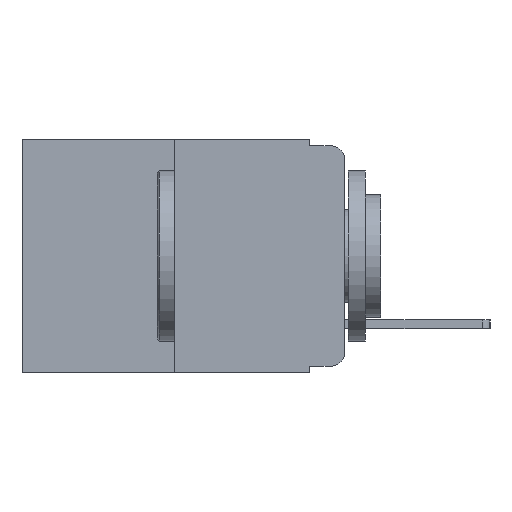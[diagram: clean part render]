
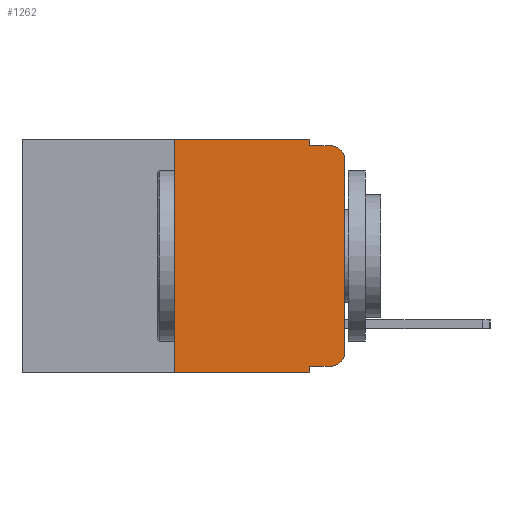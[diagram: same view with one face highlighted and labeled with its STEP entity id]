
A CAD part, left-side view. The second image highlights one B-rep face of the part: STEP entity #1262.
In plain terms, the highlighted planar face has unit normal (-1, 0, 0).
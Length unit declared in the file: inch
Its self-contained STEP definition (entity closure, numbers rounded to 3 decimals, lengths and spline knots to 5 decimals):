
#20 = CARTESIAN_POINT ( 'NONE',  ( 0., 0.02, -0.313 ) ) ;
#43 = CARTESIAN_POINT ( 'NONE',  ( 0., 0.473, 0. ) ) ;
#132 = DIRECTION ( 'NONE',  ( 0., 0., -1. ) ) ;
#146 = DIRECTION ( 'NONE',  ( -1., 0., 0. ) ) ;
#614 = VERTEX_POINT ( 'NONE', #5338 ) ;
#762 = VECTOR ( 'NONE', #6290, 39.37008 ) ;
#983 = DIRECTION ( 'NONE',  ( 1., 0., 0. ) ) ;
#1009 = DIRECTION ( 'NONE',  ( -1., 0., 0. ) ) ;
#1050 = VERTEX_POINT ( 'NONE', #8273 ) ;
#1262 = ADVANCED_FACE ( 'NONE', ( #10890 ), #2501, .F. ) ;
#1460 = AXIS2_PLACEMENT_3D ( 'NONE', #43, #983, #4947 ) ;
#1658 = EDGE_LOOP ( 'NONE', ( #9167, #11796, #8768, #2492, #11808, #3824, #4526, #4978, #3486, #3122 ) ) ;
#1795 = LINE ( 'NONE', #5846, #8770 ) ;
#1812 = CARTESIAN_POINT ( 'NONE',  ( 0., 0.02, -0.03 ) ) ;
#2006 = DIRECTION ( 'NONE',  ( 0., 0., -1. ) ) ;
#2468 = VERTEX_POINT ( 'NONE', #4721 ) ;
#2492 = ORIENTED_EDGE ( 'NONE', *, *, #7281, .F. ) ;
#2501 = PLANE ( 'NONE',  #1460 ) ;
#2860 = VECTOR ( 'NONE', #7734, 39.37008 ) ;
#2915 = VERTEX_POINT ( 'NONE', #3275 ) ;
#3122 = ORIENTED_EDGE ( 'NONE', *, *, #3303, .T. ) ;
#3126 = LINE ( 'NONE', #6664, #8311 ) ;
#3275 = CARTESIAN_POINT ( 'NONE',  ( 0., 0.02, -0.333 ) ) ;
#3303 = EDGE_CURVE ( 'NONE', #2915, #5282, #5504, .T. ) ;
#3486 = ORIENTED_EDGE ( 'NONE', *, *, #4000, .T. ) ;
#3824 = ORIENTED_EDGE ( 'NONE', *, *, #6668, .F. ) ;
#3843 = VECTOR ( 'NONE', #8742, 39.37008 ) ;
#3884 = VECTOR ( 'NONE', #4581, 39.37008 ) ;
#4000 = EDGE_CURVE ( 'NONE', #6043, #2915, #3126, .T. ) ;
#4044 = VERTEX_POINT ( 'NONE', #4362 ) ;
#4252 = CARTESIAN_POINT ( 'NONE',  ( 0., 0., -0.03 ) ) ;
#4362 = CARTESIAN_POINT ( 'NONE',  ( 0., 0.25, -0.343 ) ) ;
#4397 = VECTOR ( 'NONE', #8356, 39.37008 ) ;
#4526 = ORIENTED_EDGE ( 'NONE', *, *, #11820, .T. ) ;
#4581 = DIRECTION ( 'NONE',  ( 0., 0., -1. ) ) ;
#4705 = LINE ( 'NONE', #9235, #4397 ) ;
#4721 = CARTESIAN_POINT ( 'NONE',  ( 0., 0.25, 0. ) ) ;
#4947 = DIRECTION ( 'NONE',  ( 0., 0., -1. ) ) ;
#4978 = ORIENTED_EDGE ( 'NONE', *, *, #6020, .F. ) ;
#5108 = VERTEX_POINT ( 'NONE', #9586 ) ;
#5282 = VERTEX_POINT ( 'NONE', #11038 ) ;
#5338 = CARTESIAN_POINT ( 'NONE',  ( 0., 0.02, -0.01 ) ) ;
#5504 = CIRCLE ( 'NONE', #9614, 0.02 ) ;
#5846 = CARTESIAN_POINT ( 'NONE',  ( 0., 0.051, -0.01 ) ) ;
#6008 = CARTESIAN_POINT ( 'NONE',  ( 0., 0., 0. ) ) ;
#6020 = EDGE_CURVE ( 'NONE', #6043, #11010, #11313, .T. ) ;
#6043 = VERTEX_POINT ( 'NONE', #8791 ) ;
#6171 = LINE ( 'NONE', #6008, #8079 ) ;
#6290 = DIRECTION ( 'NONE',  ( 0., 0., 1. ) ) ;
#6315 = CARTESIAN_POINT ( 'NONE',  ( 0., 0.25, 0. ) ) ;
#6518 = LINE ( 'NONE', #10862, #3843 ) ;
#6664 = CARTESIAN_POINT ( 'NONE',  ( 0., 0.051, -0.333 ) ) ;
#6668 = EDGE_CURVE ( 'NONE', #4044, #2468, #6678, .T. ) ;
#6678 = LINE ( 'NONE', #6315, #762 ) ;
#6972 = EDGE_CURVE ( 'NONE', #2468, #1050, #8098, .T. ) ;
#7281 = EDGE_CURVE ( 'NONE', #1050, #5108, #6518, .T. ) ;
#7734 = DIRECTION ( 'NONE',  ( 0., -1., 0. ) ) ;
#7745 = CARTESIAN_POINT ( 'NONE',  ( 0., 0.473, 0. ) ) ;
#7897 = EDGE_CURVE ( 'NONE', #5108, #614, #1795, .T. ) ;
#7939 = DIRECTION ( 'NONE',  ( 0., -1., 0. ) ) ;
#8079 = VECTOR ( 'NONE', #10563, 39.37008 ) ;
#8098 = LINE ( 'NONE', #7745, #2860 ) ;
#8273 = CARTESIAN_POINT ( 'NONE',  ( 0., 0.051, 0. ) ) ;
#8311 = VECTOR ( 'NONE', #12294, 39.37008 ) ;
#8356 = DIRECTION ( 'NONE',  ( 0., -1., 0. ) ) ;
#8504 = EDGE_CURVE ( 'NONE', #9288, #614, #10461, .T. ) ;
#8742 = DIRECTION ( 'NONE',  ( 0., 0., -1. ) ) ;
#8768 = ORIENTED_EDGE ( 'NONE', *, *, #7897, .F. ) ;
#8770 = VECTOR ( 'NONE', #7939, 39.37008 ) ;
#8791 = CARTESIAN_POINT ( 'NONE',  ( 0., 0.051, -0.333 ) ) ;
#9082 = EDGE_CURVE ( 'NONE', #5282, #9288, #6171, .T. ) ;
#9167 = ORIENTED_EDGE ( 'NONE', *, *, #9082, .T. ) ;
#9235 = CARTESIAN_POINT ( 'NONE',  ( 0., 0.473, -0.343 ) ) ;
#9288 = VERTEX_POINT ( 'NONE', #4252 ) ;
#9586 = CARTESIAN_POINT ( 'NONE',  ( 0., 0.051, -0.01 ) ) ;
#9614 = AXIS2_PLACEMENT_3D ( 'NONE', #20, #146, #132 ) ;
#10461 = CIRCLE ( 'NONE', #11141, 0.02 ) ;
#10563 = DIRECTION ( 'NONE',  ( 0., 0., 1. ) ) ;
#10862 = CARTESIAN_POINT ( 'NONE',  ( 0., 0.051, 0. ) ) ;
#10890 = FACE_OUTER_BOUND ( 'NONE', #1658, .T. ) ;
#11010 = VERTEX_POINT ( 'NONE', #12202 ) ;
#11038 = CARTESIAN_POINT ( 'NONE',  ( 0., 0., -0.313 ) ) ;
#11141 = AXIS2_PLACEMENT_3D ( 'NONE', #1812, #1009, #2006 ) ;
#11313 = LINE ( 'NONE', #11486, #3884 ) ;
#11486 = CARTESIAN_POINT ( 'NONE',  ( 0., 0.051, 0. ) ) ;
#11796 = ORIENTED_EDGE ( 'NONE', *, *, #8504, .T. ) ;
#11808 = ORIENTED_EDGE ( 'NONE', *, *, #6972, .F. ) ;
#11820 = EDGE_CURVE ( 'NONE', #4044, #11010, #4705, .T. ) ;
#12202 = CARTESIAN_POINT ( 'NONE',  ( 0., 0.051, -0.343 ) ) ;
#12294 = DIRECTION ( 'NONE',  ( 0., -1., 0. ) ) ;
